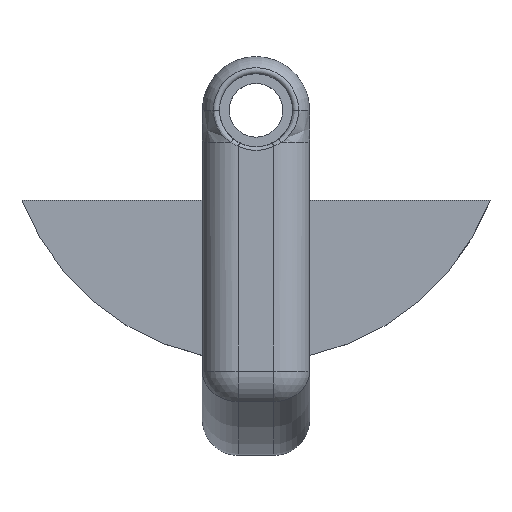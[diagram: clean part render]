
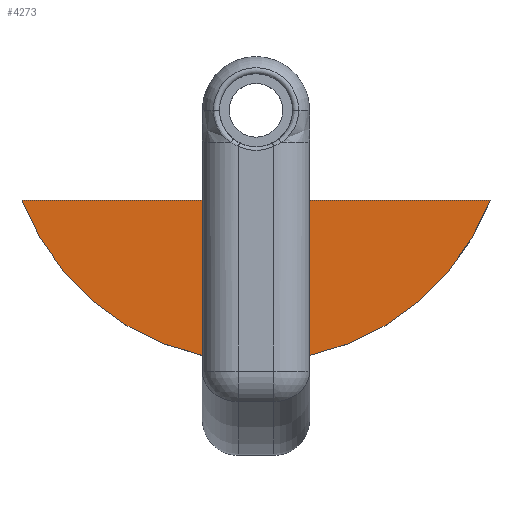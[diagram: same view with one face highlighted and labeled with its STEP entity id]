
A CAD part, top view. The second image highlights one B-rep face of the part: STEP entity #4273.
In plain terms, the highlighted planar face has unit normal (0, 0, 1).
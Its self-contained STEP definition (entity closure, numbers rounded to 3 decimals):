
#32 = VECTOR ( 'NONE', #2766, 1000. ) ;
#42 = VERTEX_POINT ( 'NONE', #4011 ) ;
#79 = CARTESIAN_POINT ( 'NONE',  ( 0., 0., 20. ) ) ;
#100 = VERTEX_POINT ( 'NONE', #2502 ) ;
#151 = LINE ( 'NONE', #79, #32 ) ;
#201 = EDGE_CURVE ( 'NONE', #3432, #2644, #2675, .T. ) ;
#237 = EDGE_CURVE ( 'NONE', #2644, #251, #2724, .T. ) ;
#251 = VERTEX_POINT ( 'NONE', #4454 ) ;
#483 = CARTESIAN_POINT ( 'NONE',  ( 20., 2.5, 20. ) ) ;
#496 = CARTESIAN_POINT ( 'NONE',  ( 2.5, -13.174, 20. ) ) ;
#536 = CIRCLE ( 'NONE', #2801, 2.5 ) ;
#586 = VECTOR ( 'NONE', #1697, 1000. ) ;
#637 = EDGE_CURVE ( 'NONE', #100, #4662, #1826, .T. ) ;
#678 = EDGE_LOOP ( 'NONE', ( #4501, #3919, #3346, #4555, #2624, #2641, #1982, #1769 ) ) ;
#787 = DIRECTION ( 'NONE',  ( -1., 0., 0. ) ) ;
#798 = CARTESIAN_POINT ( 'NONE',  ( 12.5, -13.174, 20. ) ) ;
#913 = DIRECTION ( 'NONE',  ( 1., 0., 0. ) ) ;
#930 = CIRCLE ( 'NONE', #3493, 35. ) ;
#945 = CARTESIAN_POINT ( 'NONE',  ( 0., -13.174, 20. ) ) ;
#1002 = EDGE_CURVE ( 'NONE', #4662, #42, #1058, .T. ) ;
#1058 = LINE ( 'NONE', #3380, #1075 ) ;
#1069 = EDGE_CURVE ( 'NONE', #42, #3559, #930, .T. ) ;
#1075 = VECTOR ( 'NONE', #787, 1000. ) ;
#1220 = DIRECTION ( 'NONE',  ( 1., 0., 0. ) ) ;
#1245 = CARTESIAN_POINT ( 'NONE',  ( 0., -9.187, 20. ) ) ;
#1254 = EDGE_CURVE ( 'NONE', #3076, #3432, #536, .T. ) ;
#1445 = CARTESIAN_POINT ( 'NONE',  ( 7.5, 25., 20. ) ) ;
#1488 = EDGE_CURVE ( 'NONE', #3559, #3076, #151, .T. ) ;
#1490 = DIRECTION ( 'NONE',  ( 0., 0., 1. ) ) ;
#1565 = AXIS2_PLACEMENT_3D ( 'NONE', #1445, #3943, #1841 ) ;
#1697 = DIRECTION ( 'NONE',  ( 0., -1., 0. ) ) ;
#1769 = ORIENTED_EDGE ( 'NONE', *, *, #237, .T. ) ;
#1804 = DIRECTION ( 'NONE',  ( 0., 0., 1. ) ) ;
#1826 = CIRCLE ( 'NONE', #4375, 35. ) ;
#1841 = DIRECTION ( 'NONE',  ( 1., 0., 0. ) ) ;
#1982 = ORIENTED_EDGE ( 'NONE', *, *, #201, .T. ) ;
#2093 = DIRECTION ( 'NONE',  ( 1., 0., 0. ) ) ;
#2502 = CARTESIAN_POINT ( 'NONE',  ( 15., -9.187, 20. ) ) ;
#2556 = FACE_OUTER_BOUND ( 'NONE', #678, .T. ) ;
#2624 = ORIENTED_EDGE ( 'NONE', *, *, #1488, .T. ) ;
#2641 = ORIENTED_EDGE ( 'NONE', *, *, #1254, .T. ) ;
#2644 = VERTEX_POINT ( 'NONE', #3702 ) ;
#2675 = CIRCLE ( 'NONE', #1565, 36. ) ;
#2724 = CIRCLE ( 'NONE', #4404, 2.5 ) ;
#2766 = DIRECTION ( 'NONE',  ( 0., -1., 0. ) ) ;
#2801 = AXIS2_PLACEMENT_3D ( 'NONE', #496, #3110, #913 ) ;
#3076 = VERTEX_POINT ( 'NONE', #945 ) ;
#3080 = CARTESIAN_POINT ( 'NONE',  ( 15., 0., 20. ) ) ;
#3110 = DIRECTION ( 'NONE',  ( 0., 0., -1. ) ) ;
#3247 = AXIS2_PLACEMENT_3D ( 'NONE', #483, #4197, #2093 ) ;
#3346 = ORIENTED_EDGE ( 'NONE', *, *, #1002, .T. ) ;
#3380 = CARTESIAN_POINT ( 'NONE',  ( 22.5, 12.5, 20. ) ) ;
#3387 = DIRECTION ( 'NONE',  ( 0., 0., -1. ) ) ;
#3432 = VERTEX_POINT ( 'NONE', #4393 ) ;
#3493 = AXIS2_PLACEMENT_3D ( 'NONE', #3614, #1490, #3976 ) ;
#3559 = VERTEX_POINT ( 'NONE', #1245 ) ;
#3614 = CARTESIAN_POINT ( 'NONE',  ( 7.5, 25., 20. ) ) ;
#3629 = EDGE_CURVE ( 'NONE', #100, #251, #4596, .T. ) ;
#3702 = CARTESIAN_POINT ( 'NONE',  ( 12.175, -10.695, 20. ) ) ;
#3839 = PLANE ( 'NONE',  #3247 ) ;
#3908 = CARTESIAN_POINT ( 'NONE',  ( 7.5, 25., 20. ) ) ;
#3919 = ORIENTED_EDGE ( 'NONE', *, *, #637, .T. ) ;
#3943 = DIRECTION ( 'NONE',  ( 0., 0., 1. ) ) ;
#3976 = DIRECTION ( 'NONE',  ( 1., 0., 0. ) ) ;
#4011 = CARTESIAN_POINT ( 'NONE',  ( -25.192, 12.5, 20. ) ) ;
#4197 = DIRECTION ( 'NONE',  ( 0., 0., 1. ) ) ;
#4257 = DIRECTION ( 'NONE',  ( 1., 0., 0. ) ) ;
#4273 = ADVANCED_FACE ( 'NONE', ( #2556 ), #3839, .T. ) ;
#4375 = AXIS2_PLACEMENT_3D ( 'NONE', #3908, #1804, #4257 ) ;
#4393 = CARTESIAN_POINT ( 'NONE',  ( 2.825, -10.695, 20. ) ) ;
#4404 = AXIS2_PLACEMENT_3D ( 'NONE', #798, #3387, #1220 ) ;
#4454 = CARTESIAN_POINT ( 'NONE',  ( 15., -13.174, 20. ) ) ;
#4501 = ORIENTED_EDGE ( 'NONE', *, *, #3629, .F. ) ;
#4555 = ORIENTED_EDGE ( 'NONE', *, *, #1069, .T. ) ;
#4582 = CARTESIAN_POINT ( 'NONE',  ( 40.192, 12.5, 20. ) ) ;
#4596 = LINE ( 'NONE', #3080, #586 ) ;
#4662 = VERTEX_POINT ( 'NONE', #4582 ) ;
